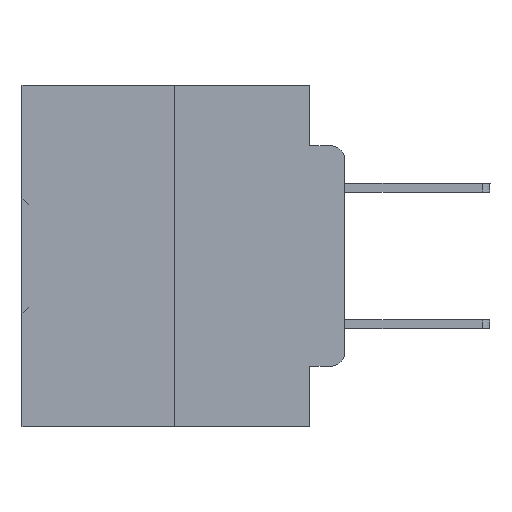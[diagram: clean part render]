
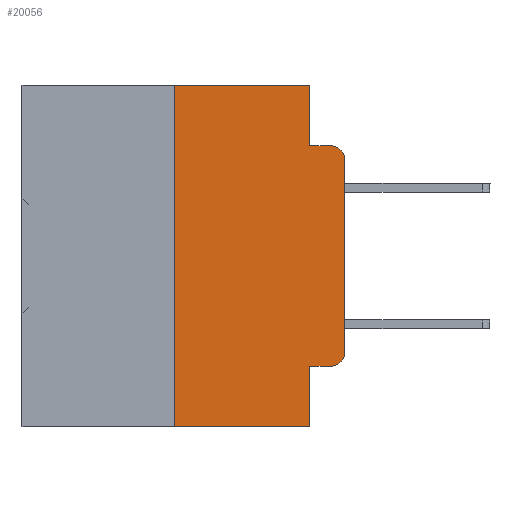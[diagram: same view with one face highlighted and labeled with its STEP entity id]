
A CAD part, left-side view. The second image highlights one B-rep face of the part: STEP entity #20056.
In plain terms, the highlighted planar face has unit normal (-1, 0, 0).
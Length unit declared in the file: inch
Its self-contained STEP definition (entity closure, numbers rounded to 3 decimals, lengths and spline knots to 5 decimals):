
#1046 = LINE ( 'NONE', #20379, #23850 ) ;
#1146 = CARTESIAN_POINT ( 'NONE',  ( 0., 0.02, -0.3915 ) ) ;
#2213 = VECTOR ( 'NONE', #31476, 39.37008 ) ;
#2214 = VERTEX_POINT ( 'NONE', #37887 ) ;
#2723 = CARTESIAN_POINT ( 'NONE',  ( 0., 0.473, -0.5 ) ) ;
#2980 = DIRECTION ( 'NONE',  ( 0., -1., 0. ) ) ;
#3078 = ORIENTED_EDGE ( 'NONE', *, *, #28233, .T. ) ;
#3128 = CARTESIAN_POINT ( 'NONE',  ( 0., 0.473, 0. ) ) ;
#3203 = VECTOR ( 'NONE', #14600, 39.37008 ) ;
#3756 = CARTESIAN_POINT ( 'NONE',  ( 0., 0.051, -0.4115 ) ) ;
#4381 = LINE ( 'NONE', #16453, #36020 ) ;
#4897 = CARTESIAN_POINT ( 'NONE',  ( 0., 0.25, 0. ) ) ;
#4951 = VERTEX_POINT ( 'NONE', #10422 ) ;
#5119 = CARTESIAN_POINT ( 'NONE',  ( 0., 0., 0. ) ) ;
#5916 = VECTOR ( 'NONE', #2980, 39.37008 ) ;
#6275 = VERTEX_POINT ( 'NONE', #25076 ) ;
#8111 = EDGE_CURVE ( 'NONE', #12405, #4951, #34252, .T. ) ;
#8148 = CARTESIAN_POINT ( 'NONE',  ( 0., 0., -0.1085 ) ) ;
#8264 = CIRCLE ( 'NONE', #30655, 0.02 ) ;
#8347 = VECTOR ( 'NONE', #24547, 39.37008 ) ;
#8521 = DIRECTION ( 'NONE',  ( 0., -1., 0. ) ) ;
#8963 = DIRECTION ( 'NONE',  ( 1., 0., 0. ) ) ;
#9438 = VERTEX_POINT ( 'NONE', #4897 ) ;
#9756 = CARTESIAN_POINT ( 'NONE',  ( 0., 0.051, 0. ) ) ;
#10393 = ORIENTED_EDGE ( 'NONE', *, *, #36267, .F. ) ;
#10422 = CARTESIAN_POINT ( 'NONE',  ( 0., 0., -0.3915 ) ) ;
#11206 = DIRECTION ( 'NONE',  ( -1., 0., 0. ) ) ;
#11322 = EDGE_LOOP ( 'NONE', ( #16235, #3078, #14335, #18524, #25985, #10393, #27059, #30341, #35708, #31951 ) ) ;
#12130 = EDGE_CURVE ( 'NONE', #9438, #24148, #1046, .T. ) ;
#12405 = VERTEX_POINT ( 'NONE', #22036 ) ;
#12757 = DIRECTION ( 'NONE',  ( 0., 0., -1. ) ) ;
#13572 = DIRECTION ( 'NONE',  ( 0., -1., 0. ) ) ;
#13926 = CARTESIAN_POINT ( 'NONE',  ( 0., 0.02, -0.1085 ) ) ;
#13964 = VERTEX_POINT ( 'NONE', #32411 ) ;
#14335 = ORIENTED_EDGE ( 'NONE', *, *, #38018, .F. ) ;
#14600 = DIRECTION ( 'NONE',  ( 0., 0., 1. ) ) ;
#15836 = LINE ( 'NONE', #3756, #8347 ) ;
#16235 = ORIENTED_EDGE ( 'NONE', *, *, #35392, .T. ) ;
#16274 = VERTEX_POINT ( 'NONE', #32214 ) ;
#16453 = CARTESIAN_POINT ( 'NONE',  ( 0., 0.051, -0.0885 ) ) ;
#17152 = LINE ( 'NONE', #5119, #3203 ) ;
#17711 = VERTEX_POINT ( 'NONE', #21751 ) ;
#18331 = PLANE ( 'NONE',  #37231 ) ;
#18515 = VERTEX_POINT ( 'NONE', #8148 ) ;
#18524 = ORIENTED_EDGE ( 'NONE', *, *, #36455, .F. ) ;
#18647 = CARTESIAN_POINT ( 'NONE',  ( 0., 0.051, 0. ) ) ;
#19208 = DIRECTION ( 'NONE',  ( 0., 0., -1. ) ) ;
#19439 = CARTESIAN_POINT ( 'NONE',  ( 0., 0.25, 0. ) ) ;
#20056 = ADVANCED_FACE ( 'NONE', ( #25011 ), #18331, .F. ) ;
#20379 = CARTESIAN_POINT ( 'NONE',  ( 0., 0.473, 0. ) ) ;
#21264 = VECTOR ( 'NONE', #21396, 39.37008 ) ;
#21396 = DIRECTION ( 'NONE',  ( 0., 0., -1. ) ) ;
#21751 = CARTESIAN_POINT ( 'NONE',  ( 0., 0.25, -0.5 ) ) ;
#21932 = EDGE_CURVE ( 'NONE', #2214, #13964, #26741, .T. ) ;
#22036 = CARTESIAN_POINT ( 'NONE',  ( 0., 0.02, -0.4115 ) ) ;
#22662 = LINE ( 'NONE', #2723, #5916 ) ;
#23850 = VECTOR ( 'NONE', #8521, 39.37008 ) ;
#23941 = DIRECTION ( 'NONE',  ( 0., 0., -1. ) ) ;
#23975 = VECTOR ( 'NONE', #12757, 39.37008 ) ;
#24148 = VERTEX_POINT ( 'NONE', #35636 ) ;
#24547 = DIRECTION ( 'NONE',  ( 0., -1., 0. ) ) ;
#24840 = EDGE_CURVE ( 'NONE', #2214, #12405, #15836, .T. ) ;
#25011 = FACE_OUTER_BOUND ( 'NONE', #11322, .T. ) ;
#25076 = CARTESIAN_POINT ( 'NONE',  ( 0., 0.02, -0.0885 ) ) ;
#25985 = ORIENTED_EDGE ( 'NONE', *, *, #12130, .F. ) ;
#26725 = EDGE_CURVE ( 'NONE', #17711, #13964, #22662, .T. ) ;
#26741 = LINE ( 'NONE', #9756, #23975 ) ;
#27059 = ORIENTED_EDGE ( 'NONE', *, *, #26725, .T. ) ;
#27301 = LINE ( 'NONE', #19439, #2213 ) ;
#28233 = EDGE_CURVE ( 'NONE', #18515, #6275, #8264, .T. ) ;
#28844 = DIRECTION ( 'NONE',  ( 0., 0., -1. ) ) ;
#30341 = ORIENTED_EDGE ( 'NONE', *, *, #21932, .F. ) ;
#30655 = AXIS2_PLACEMENT_3D ( 'NONE', #13926, #11206, #28844 ) ;
#30666 = AXIS2_PLACEMENT_3D ( 'NONE', #1146, #36984, #19208 ) ;
#31476 = DIRECTION ( 'NONE',  ( 0., 0., 1. ) ) ;
#31951 = ORIENTED_EDGE ( 'NONE', *, *, #8111, .T. ) ;
#32214 = CARTESIAN_POINT ( 'NONE',  ( 0., 0.051, -0.0885 ) ) ;
#32411 = CARTESIAN_POINT ( 'NONE',  ( 0., 0.051, -0.5 ) ) ;
#33771 = LINE ( 'NONE', #18647, #21264 ) ;
#34252 = CIRCLE ( 'NONE', #30666, 0.02 ) ;
#35392 = EDGE_CURVE ( 'NONE', #4951, #18515, #17152, .T. ) ;
#35636 = CARTESIAN_POINT ( 'NONE',  ( 0., 0.051, 0. ) ) ;
#35708 = ORIENTED_EDGE ( 'NONE', *, *, #24840, .T. ) ;
#36020 = VECTOR ( 'NONE', #13572, 39.37008 ) ;
#36267 = EDGE_CURVE ( 'NONE', #17711, #9438, #27301, .T. ) ;
#36455 = EDGE_CURVE ( 'NONE', #24148, #16274, #33771, .T. ) ;
#36984 = DIRECTION ( 'NONE',  ( -1., 0., 0. ) ) ;
#37231 = AXIS2_PLACEMENT_3D ( 'NONE', #3128, #8963, #23941 ) ;
#37887 = CARTESIAN_POINT ( 'NONE',  ( 0., 0.051, -0.4115 ) ) ;
#38018 = EDGE_CURVE ( 'NONE', #16274, #6275, #4381, .T. ) ;
